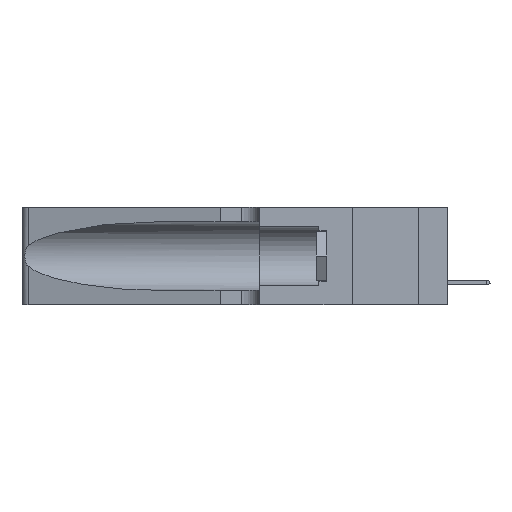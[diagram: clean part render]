
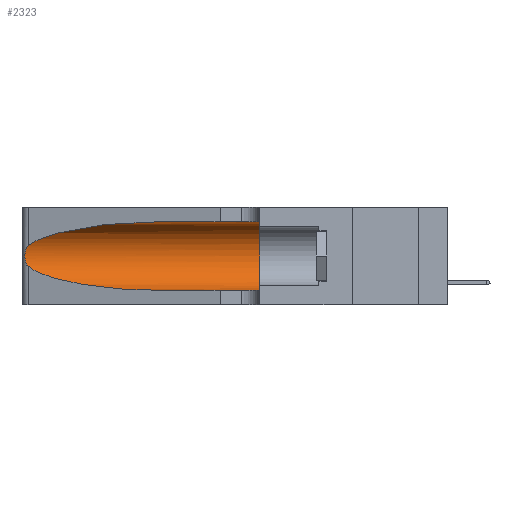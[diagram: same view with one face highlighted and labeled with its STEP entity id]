
A CAD part, left-side view. The second image highlights one B-rep face of the part: STEP entity #2323.
In plain terms, the highlighted cylindrical face has radius 3.308 mm (diameter 6.617 mm), a partial arc.
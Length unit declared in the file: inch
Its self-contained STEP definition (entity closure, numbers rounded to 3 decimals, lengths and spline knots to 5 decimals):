
#145 = EDGE_CURVE ( 'NONE', #1416, #8144, #7001, .T. ) ;
#358 = AXIS2_PLACEMENT_3D ( 'NONE', #26369, #20220, #22093 ) ;
#602 = CARTESIAN_POINT ( 'NONE',  ( 0.25639, 1.23184, 0.21858 ) ) ;
#694 = CARTESIAN_POINT ( 'NONE',  ( 0.25487, 1.22718, 0.22369 ) ) ;
#714 = CARTESIAN_POINT ( 'NONE',  ( 0.1305, 0.35, 0.31525 ) ) ;
#791 = CARTESIAN_POINT ( 'NONE',  ( 0.26075, 1.23896, 0.19203 ) ) ;
#1416 = VERTEX_POINT ( 'NONE', #714 ) ;
#1466 = DIRECTION ( 'NONE',  ( 0., -1., 0. ) ) ;
#1744 = CARTESIAN_POINT ( 'NONE',  ( 0.1305, 0.72297, 0.05475 ) ) ;
#1850 = CARTESIAN_POINT ( 'NONE',  ( 0.18966, 0.96281, 0.05475 ) ) ;
#2323 = ADVANCED_FACE ( 'NONE', ( #19306 ), #7544, .F. ) ;
#2938 = CARTESIAN_POINT ( 'NONE',  ( 0.25487, 1.22718, 0.22369 ) ) ;
#3423 = EDGE_LOOP ( 'NONE', ( #19831, #24877, #5184, #16626, #7024, #7529 ) ) ;
#3568 = VECTOR ( 'NONE', #20542, 39.37008 ) ;
#4179 = CARTESIAN_POINT ( 'NONE',  ( 0.25487, 1.22718, 0.14631 ) ) ;
#4473 = EDGE_CURVE ( 'NONE', #7726, #15372, #13716, .T. ) ;
#4834 = CARTESIAN_POINT ( 'NONE',  ( 0.26017, 1.23833, 0.17102 ) ) ;
#5109 = CARTESIAN_POINT ( 'NONE',  ( 0.25639, 1.23186, 0.15144 ) ) ;
#5184 = ORIENTED_EDGE ( 'NONE', *, *, #17690, .T. ) ;
#5756 = CARTESIAN_POINT ( 'NONE',  ( 0.1305, 1.61858, 0.31525 ) ) ;
#6045 = EDGE_CURVE ( 'NONE', #8800, #8144, #20060, .T. ) ;
#7001 = CIRCLE ( 'NONE', #358, 0.13025 ) ;
#7024 = ORIENTED_EDGE ( 'NONE', *, *, #145, .F. ) ;
#7180 = CARTESIAN_POINT ( 'NONE',  ( 0.25555, 1.22994, 0.2215 ) ) ;
#7342 = CARTESIAN_POINT ( 'NONE',  ( 0.18966, 0.96281, 0.31525 ) ) ;
#7529 = ORIENTED_EDGE ( 'NONE', *, *, #9498, .F. ) ;
#7544 = CYLINDRICAL_SURFACE ( 'NONE', #13023, 0.13025 ) ;
#7726 = VERTEX_POINT ( 'NONE', #21879 ) ;
#8144 = VERTEX_POINT ( 'NONE', #10260 ) ;
#8800 = VERTEX_POINT ( 'NONE', #1744 ) ;
#9163 = CARTESIAN_POINT ( 'NONE',  ( 0.25854, 1.2359, 0.20912 ) ) ;
#9358 = CARTESIAN_POINT ( 'NONE',  ( 0.26075, 1.23896, 0.178 ) ) ;
#9498 = EDGE_CURVE ( 'NONE', #7726, #1416, #10460, .T. ) ;
#10260 = CARTESIAN_POINT ( 'NONE',  ( 0.1305, 0.35, 0.05475 ) ) ;
#10460 = LINE ( 'NONE', #5756, #21216 ) ;
#11529 = CARTESIAN_POINT ( 'NONE',  ( 0.26018, 1.23835, 0.19895 ) ) ;
#12428 = VERTEX_POINT ( 'NONE', #16545 ) ;
#13023 = AXIS2_PLACEMENT_3D ( 'NONE', #18220, #24591, #20383 ) ;
#13473 = CARTESIAN_POINT ( 'NONE',  ( 0.1305, 0.72297, 0.31525 ) ) ;
#13716 =( BOUNDED_CURVE ( )  B_SPLINE_CURVE ( 3, ( #13473, #7342, #22494, #2938 ),
 .UNSPECIFIED., .F., .F. ) 
 B_SPLINE_CURVE_WITH_KNOTS ( ( 4, 4 ),
 ( 1.5708, 2.84003 ),
 .UNSPECIFIED. ) 
 CURVE ( )  GEOMETRIC_REPRESENTATION_ITEM ( )  RATIONAL_B_SPLINE_CURVE ( ( 1., 0.87, 0.87, 1. ) ) 
 REPRESENTATION_ITEM ( '' )  );
#15372 = VERTEX_POINT ( 'NONE', #20268 ) ;
#16545 = CARTESIAN_POINT ( 'NONE',  ( 0.25487, 1.22718, 0.14631 ) ) ;
#16626 = ORIENTED_EDGE ( 'NONE', *, *, #6045, .T. ) ;
#17327 = B_SPLINE_CURVE_WITH_KNOTS ( 'NONE', 3,
 ( #694, #7180, #602, #17823, #9163, #11529, #791, #9358, #4834, #19882, #18005, #5109, #24195, #20174 ),
 .UNSPECIFIED., .F., .F.,
 ( 4, 2, 2, 2, 2, 2, 4 ),
 ( 0., 0.00027, 0.00053, 0.00107, 0.0016, 0.00187, 0.00214 ),
 .UNSPECIFIED. ) ;
#17690 = EDGE_CURVE ( 'NONE', #12428, #8800, #19552, .T. ) ;
#17823 = CARTESIAN_POINT ( 'NONE',  ( 0.25787, 1.23484, 0.2124 ) ) ;
#18005 = CARTESIAN_POINT ( 'NONE',  ( 0.25789, 1.23486, 0.15765 ) ) ;
#18220 = CARTESIAN_POINT ( 'NONE',  ( 0.1305, 1.61858, 0.185 ) ) ;
#19306 = FACE_OUTER_BOUND ( 'NONE', #3423, .T. ) ;
#19552 =( BOUNDED_CURVE ( )  B_SPLINE_CURVE ( 3, ( #4179, #27545, #1850, #25513 ),
 .UNSPECIFIED., .F., .F. ) 
 B_SPLINE_CURVE_WITH_KNOTS ( ( 4, 4 ),
 ( 3.44316, 4.71239 ),
 .UNSPECIFIED. ) 
 CURVE ( )  GEOMETRIC_REPRESENTATION_ITEM ( )  RATIONAL_B_SPLINE_CURVE ( ( 1., 0.87, 0.87, 1. ) ) 
 REPRESENTATION_ITEM ( '' )  );
#19831 = ORIENTED_EDGE ( 'NONE', *, *, #4473, .T. ) ;
#19882 = CARTESIAN_POINT ( 'NONE',  ( 0.25856, 1.23593, 0.16098 ) ) ;
#20060 = LINE ( 'NONE', #20340, #3568 ) ;
#20174 = CARTESIAN_POINT ( 'NONE',  ( 0.25487, 1.22718, 0.14631 ) ) ;
#20220 = DIRECTION ( 'NONE',  ( 0., 1., 0. ) ) ;
#20268 = CARTESIAN_POINT ( 'NONE',  ( 0.25487, 1.22718, 0.22369 ) ) ;
#20340 = CARTESIAN_POINT ( 'NONE',  ( 0.1305, 1.61858, 0.05475 ) ) ;
#20383 = DIRECTION ( 'NONE',  ( 0., 0., -1. ) ) ;
#20542 = DIRECTION ( 'NONE',  ( 0., -1., 0. ) ) ;
#21216 = VECTOR ( 'NONE', #1466, 39.37008 ) ;
#21879 = CARTESIAN_POINT ( 'NONE',  ( 0.1305, 0.72297, 0.31525 ) ) ;
#22093 = DIRECTION ( 'NONE',  ( 0., 0., 1. ) ) ;
#22494 = CARTESIAN_POINT ( 'NONE',  ( 0.2373, 1.15595, 0.28018 ) ) ;
#23518 = EDGE_CURVE ( 'NONE', #15372, #12428, #17327, .T. ) ;
#24195 = CARTESIAN_POINT ( 'NONE',  ( 0.25555, 1.22993, 0.14849 ) ) ;
#24591 = DIRECTION ( 'NONE',  ( 0., -1., 0. ) ) ;
#24877 = ORIENTED_EDGE ( 'NONE', *, *, #23518, .T. ) ;
#25513 = CARTESIAN_POINT ( 'NONE',  ( 0.1305, 0.72297, 0.05475 ) ) ;
#26369 = CARTESIAN_POINT ( 'NONE',  ( 0.1305, 0.35, 0.185 ) ) ;
#27545 = CARTESIAN_POINT ( 'NONE',  ( 0.2373, 1.15595, 0.08982 ) ) ;
